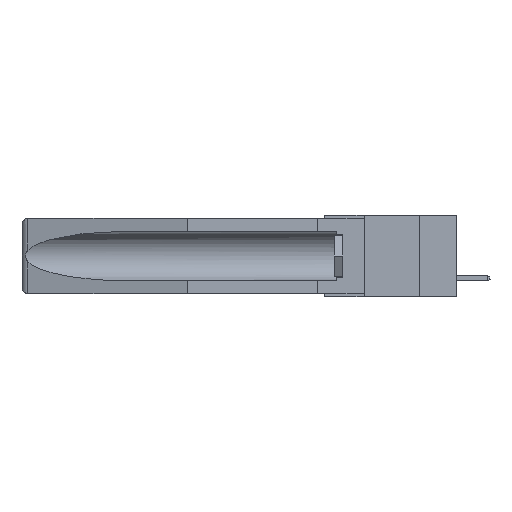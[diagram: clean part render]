
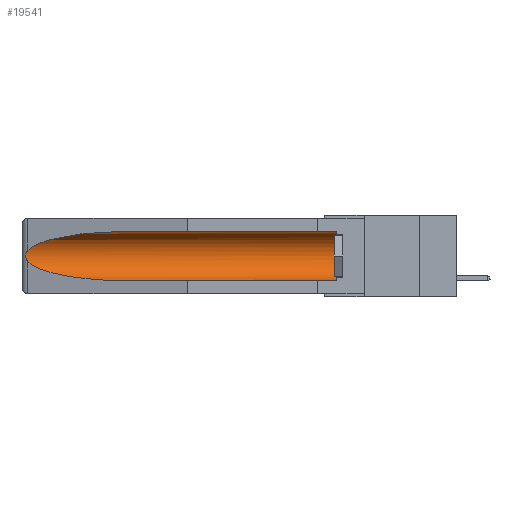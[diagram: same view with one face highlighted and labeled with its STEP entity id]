
A CAD part, left-side view. The second image highlights one B-rep face of the part: STEP entity #19541.
In plain terms, the highlighted cylindrical face has radius 2.857 mm (diameter 5.715 mm), a partial arc.
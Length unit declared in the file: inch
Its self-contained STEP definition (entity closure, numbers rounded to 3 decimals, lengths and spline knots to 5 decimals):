
#261 = CARTESIAN_POINT ( 'NONE',  ( 0.155, -0.30754, -0.059 ) ) ;
#535 = CARTESIAN_POINT ( 'NONE',  ( 0.21114, 1.30732, -0.284 ) ) ;
#817 = CARTESIAN_POINT ( 'NONE',  ( 0.26597, 1.5296, -0.19026 ) ) ;
#838 = EDGE_LOOP ( 'NONE', ( #14359, #3288, #22718, #19269, #7480, #14370 ) ) ;
#891 = CARTESIAN_POINT ( 'NONE',  ( 0.26597, 1.52961, -0.15275 ) ) ;
#977 = LINE ( 'NONE', #16155, #17501 ) ;
#2105 = VERTEX_POINT ( 'NONE', #2310 ) ;
#2149 = CARTESIAN_POINT ( 'NONE',  ( 0.25451, 1.48313, -0.24835 ) ) ;
#2310 = CARTESIAN_POINT ( 'NONE',  ( 0.155, 0.126, -0.284 ) ) ;
#2369 = DIRECTION ( 'NONE',  ( 0., 1., 0. ) ) ;
#2916 = DIRECTION ( 'NONE',  ( 0., 0., 1. ) ) ;
#3288 = ORIENTED_EDGE ( 'NONE', *, *, #9672, .T. ) ;
#3397 = CARTESIAN_POINT ( 'NONE',  ( 0.26537, 1.52718, -0.14972 ) ) ;
#3796 = CARTESIAN_POINT ( 'NONE',  ( 0.155, 1.07973, -0.059 ) ) ;
#4429 = VERTEX_POINT ( 'NONE', #11544 ) ;
#4920 = EDGE_CURVE ( 'NONE', #2105, #4429, #22497, .T. ) ;
#5360 = B_SPLINE_CURVE_WITH_KNOTS ( 'NONE', 3,
 ( #20141, #891, #5960, #13186, #18300, #7726, #15002, #20060, #817, #9502 ),
 .UNSPECIFIED., .F., .F.,
 ( 4, 2, 2, 2, 4 ),
 ( 0., 0.00029, 0.00058, 0.00087, 0.00117 ),
 .UNSPECIFIED. ) ;
#5960 = CARTESIAN_POINT ( 'NONE',  ( 0.26654, 1.53092, -0.15636 ) ) ;
#6238 = CARTESIAN_POINT ( 'NONE',  ( 0.155, -0.30754, -0.1715 ) ) ;
#6553 = VECTOR ( 'NONE', #9168, 39.37008 ) ;
#7480 = ORIENTED_EDGE ( 'NONE', *, *, #4920, .T. ) ;
#7500 = CARTESIAN_POINT ( 'NONE',  ( 0.21114, 1.30732, -0.059 ) ) ;
#7565 = VERTEX_POINT ( 'NONE', #22318 ) ;
#7726 = CARTESIAN_POINT ( 'NONE',  ( 0.2675, 1.53308, -0.17534 ) ) ;
#8722 = VERTEX_POINT ( 'NONE', #10024 ) ;
#9168 = DIRECTION ( 'NONE',  ( 0., 1., 0. ) ) ;
#9294 = DIRECTION ( 'NONE',  ( 0., -1., 0. ) ) ;
#9445 = CARTESIAN_POINT ( 'NONE',  ( 0.26537, 1.52718, -0.19328 ) ) ;
#9502 = CARTESIAN_POINT ( 'NONE',  ( 0.26537, 1.52718, -0.19328 ) ) ;
#9638 = FACE_OUTER_BOUND ( 'NONE', #838, .T. ) ;
#9672 = EDGE_CURVE ( 'NONE', #15750, #8722, #5360, .T. ) ;
#10024 = CARTESIAN_POINT ( 'NONE',  ( 0.26537, 1.52718, -0.19328 ) ) ;
#10322 = EDGE_CURVE ( 'NONE', #8722, #7565, #16673, .T. ) ;
#10702 =( BOUNDED_CURVE ( )  B_SPLINE_CURVE ( 3, ( #3796, #7500, #21589, #16158 ),
 .UNSPECIFIED., .F., .F. ) 
 B_SPLINE_CURVE_WITH_KNOTS ( ( 4, 4 ),
 ( 4.71239, 6.08839 ),
 .UNSPECIFIED. ) 
 CURVE ( )  GEOMETRIC_REPRESENTATION_ITEM ( )  RATIONAL_B_SPLINE_CURVE ( ( 1., 0.848, 0.848, 1. ) ) 
 REPRESENTATION_ITEM ( '' )  );
#11225 = LINE ( 'NONE', #261, #6553 ) ;
#11390 = EDGE_CURVE ( 'NONE', #2105, #7565, #977, .T. ) ;
#11544 = CARTESIAN_POINT ( 'NONE',  ( 0.155, 0.126, -0.059 ) ) ;
#13186 = CARTESIAN_POINT ( 'NONE',  ( 0.2673, 1.5327, -0.16383 ) ) ;
#14359 = ORIENTED_EDGE ( 'NONE', *, *, #21477, .T. ) ;
#14370 = ORIENTED_EDGE ( 'NONE', *, *, #21175, .T. ) ;
#15002 = CARTESIAN_POINT ( 'NONE',  ( 0.2673, 1.53269, -0.17917 ) ) ;
#15750 = VERTEX_POINT ( 'NONE', #3397 ) ;
#16155 = CARTESIAN_POINT ( 'NONE',  ( 0.155, -0.30754, -0.284 ) ) ;
#16158 = CARTESIAN_POINT ( 'NONE',  ( 0.26537, 1.52718, -0.14972 ) ) ;
#16211 = AXIS2_PLACEMENT_3D ( 'NONE', #18170, #9294, #21604 ) ;
#16673 =( BOUNDED_CURVE ( )  B_SPLINE_CURVE ( 3, ( #9445, #2149, #535, #21678 ),
 .UNSPECIFIED., .F., .F. ) 
 B_SPLINE_CURVE_WITH_KNOTS ( ( 4, 4 ),
 ( 0.1948, 1.5708 ),
 .UNSPECIFIED. ) 
 CURVE ( )  GEOMETRIC_REPRESENTATION_ITEM ( )  RATIONAL_B_SPLINE_CURVE ( ( 1., 0.848, 0.848, 1. ) ) 
 REPRESENTATION_ITEM ( '' )  );
#17233 = VERTEX_POINT ( 'NONE', #19429 ) ;
#17501 = VECTOR ( 'NONE', #2369, 39.37008 ) ;
#18146 = AXIS2_PLACEMENT_3D ( 'NONE', #6238, #18704, #2916 ) ;
#18170 = CARTESIAN_POINT ( 'NONE',  ( 0.155, 0.126, -0.1715 ) ) ;
#18300 = CARTESIAN_POINT ( 'NONE',  ( 0.2675, 1.53308, -0.16763 ) ) ;
#18704 = DIRECTION ( 'NONE',  ( 0., 1., 0. ) ) ;
#19015 = CYLINDRICAL_SURFACE ( 'NONE', #18146, 0.1125 ) ;
#19269 = ORIENTED_EDGE ( 'NONE', *, *, #11390, .F. ) ;
#19429 = CARTESIAN_POINT ( 'NONE',  ( 0.155, 1.07973, -0.059 ) ) ;
#19541 = ADVANCED_FACE ( 'NONE', ( #9638 ), #19015, .F. ) ;
#20060 = CARTESIAN_POINT ( 'NONE',  ( 0.26655, 1.53094, -0.18657 ) ) ;
#20141 = CARTESIAN_POINT ( 'NONE',  ( 0.26537, 1.52718, -0.14972 ) ) ;
#21175 = EDGE_CURVE ( 'NONE', #4429, #17233, #11225, .T. ) ;
#21477 = EDGE_CURVE ( 'NONE', #17233, #15750, #10702, .T. ) ;
#21589 = CARTESIAN_POINT ( 'NONE',  ( 0.25451, 1.48313, -0.09465 ) ) ;
#21604 = DIRECTION ( 'NONE',  ( 0., 0., 1. ) ) ;
#21678 = CARTESIAN_POINT ( 'NONE',  ( 0.155, 1.07973, -0.284 ) ) ;
#22318 = CARTESIAN_POINT ( 'NONE',  ( 0.155, 1.07973, -0.284 ) ) ;
#22497 = CIRCLE ( 'NONE', #16211, 0.1125 ) ;
#22718 = ORIENTED_EDGE ( 'NONE', *, *, #10322, .T. ) ;
